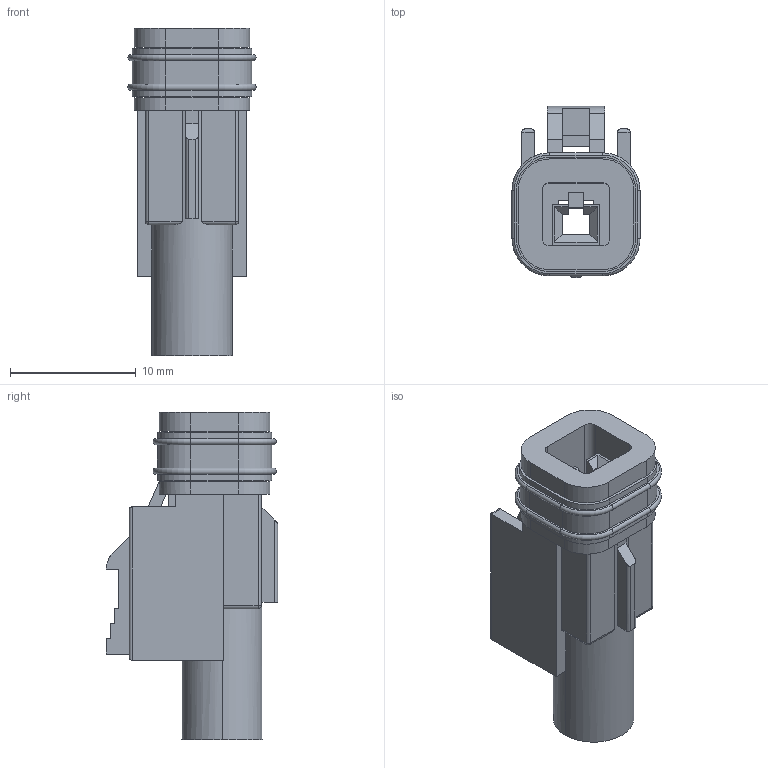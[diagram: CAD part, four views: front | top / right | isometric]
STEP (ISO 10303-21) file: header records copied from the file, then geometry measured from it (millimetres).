
FILE_DESCRIPTION (( 'STEP AP214' ), '1' );
FILE_NAME ('570-001-000-200.STEP', '2020-07-30T14:06:25', ( '' ), ( '' ), 'SwSTEP 2.0', 'SolidWorks 2020', '' );
FILE_SCHEMA (( 'AUTOMOTIVE_DESIGN' ));
Length unit declared in the file: millimetre
Products named in the file (3): 570-001-000-200_Housing; 570-001-000-200_Rubber; 570-001-000-200
Assembly tree (2 placements, depth 2):
  570-001-000-200
    570-001-000-200_Housing
    570-001-000-200_Rubber
Bounding box: 10.18 x 13.6 x 26 mm (x, y, z)
Volume: 1075.1 mm3; surface area: 2288.2 mm2
Topology: 3 solids, 3 shells, 279 faces, 751 edges, 484 vertices
Faces by surface type: plane 169, cylinder 84, torus 24, sphere 2
Entity records: 8832 total; most frequent: CARTESIAN_POINT 1583, DIRECTION 1511, ORIENTED_EDGE 1498, EDGE_CURVE 749, LINE 519, VECTOR 519, AXIS2_PLACEMENT_3D 496, VERTEX_POINT 484
